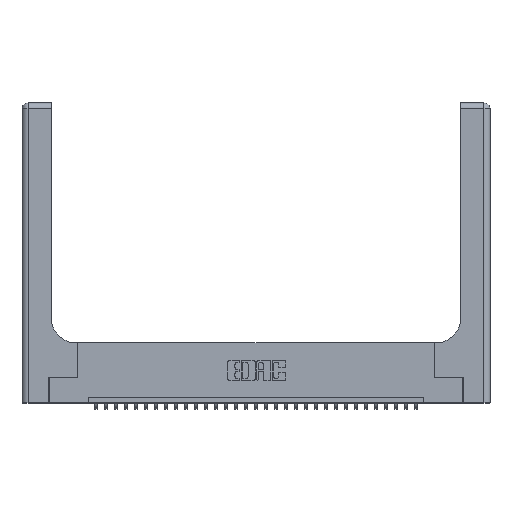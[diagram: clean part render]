
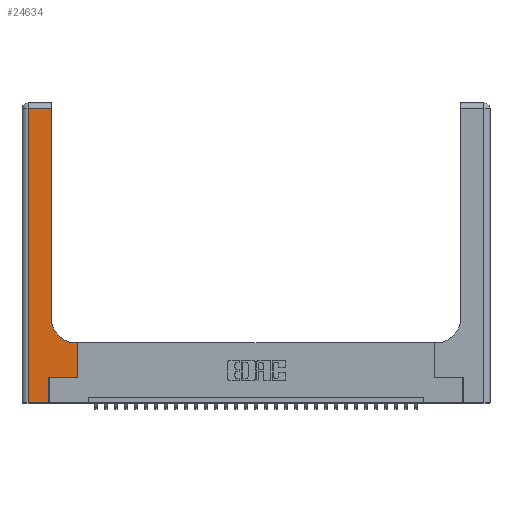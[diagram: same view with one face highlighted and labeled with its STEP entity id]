
A CAD part, top view. The second image highlights one B-rep face of the part: STEP entity #24634.
In plain terms, the highlighted planar face has unit normal (0, 0, 1).
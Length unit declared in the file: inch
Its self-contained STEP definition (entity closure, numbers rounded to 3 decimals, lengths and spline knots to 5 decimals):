
#77 = VERTEX_POINT ( 'NONE', #18571 ) ;
#371 = VECTOR ( 'NONE', #17619, 39.37008 ) ;
#860 = VECTOR ( 'NONE', #27896, 39.37008 ) ;
#1124 = LINE ( 'NONE', #12731, #371 ) ;
#2771 = VECTOR ( 'NONE', #21367, 39.37008 ) ;
#2856 = ORIENTED_EDGE ( 'NONE', *, *, #28152, .T. ) ;
#3835 = DIRECTION ( 'NONE',  ( 1., 0., 0. ) ) ;
#3898 = AXIS2_PLACEMENT_3D ( 'NONE', #25846, #25738, #23431 ) ;
#4235 = VECTOR ( 'NONE', #31249, 39.37008 ) ;
#4257 = ORIENTED_EDGE ( 'NONE', *, *, #28473, .T. ) ;
#4425 = CARTESIAN_POINT ( 'NONE',  ( 0.5415, 0.6, 0.37 ) ) ;
#5604 = ORIENTED_EDGE ( 'NONE', *, *, #16896, .T. ) ;
#5617 = AXIS2_PLACEMENT_3D ( 'NONE', #22779, #8044, #5933 ) ;
#5933 = DIRECTION ( 'NONE',  ( -1., 0., 0. ) ) ;
#6638 = ORIENTED_EDGE ( 'NONE', *, *, #18883, .T. ) ;
#7008 = LINE ( 'NONE', #28454, #16888 ) ;
#7101 = CARTESIAN_POINT ( 'NONE',  ( 0.2915, 3., 0.37 ) ) ;
#8044 = DIRECTION ( 'NONE',  ( 0., 0., -1. ) ) ;
#8745 = CARTESIAN_POINT ( 'NONE',  ( 0., 0., 0.37 ) ) ;
#9005 = ORIENTED_EDGE ( 'NONE', *, *, #16906, .T. ) ;
#9894 = LINE ( 'NONE', #28218, #2771 ) ;
#9935 = ORIENTED_EDGE ( 'NONE', *, *, #11851, .T. ) ;
#10316 = LINE ( 'NONE', #16171, #860 ) ;
#10802 = EDGE_CURVE ( 'NONE', #11875, #19676, #9894, .T. ) ;
#11637 = DIRECTION ( 'NONE',  ( 0., -1., 0. ) ) ;
#11851 = EDGE_CURVE ( 'NONE', #18672, #19126, #17059, .T. ) ;
#11875 = VERTEX_POINT ( 'NONE', #30527 ) ;
#11893 = VECTOR ( 'NONE', #11637, 39.37008 ) ;
#12731 = CARTESIAN_POINT ( 'NONE',  ( 0.5585, 0.25, 0.37 ) ) ;
#13619 = VECTOR ( 'NONE', #3835, 39.37008 ) ;
#13732 = VERTEX_POINT ( 'NONE', #4425 ) ;
#13745 = VERTEX_POINT ( 'NONE', #18265 ) ;
#13988 = DIRECTION ( 'NONE',  ( 0., 1., 0. ) ) ;
#16171 = CARTESIAN_POINT ( 'NONE',  ( 0., 2.94, 0.37 ) ) ;
#16888 = VECTOR ( 'NONE', #13988, 39.37008 ) ;
#16896 = EDGE_CURVE ( 'NONE', #19126, #11875, #7008, .T. ) ;
#16906 = EDGE_CURVE ( 'NONE', #25138, #18672, #23685, .T. ) ;
#17059 = LINE ( 'NONE', #8745, #13619 ) ;
#17619 = DIRECTION ( 'NONE',  ( 0., 1., 0. ) ) ;
#18031 = LINE ( 'NONE', #7101, #24487 ) ;
#18265 = CARTESIAN_POINT ( 'NONE',  ( 0.5585, 0.6, 0.37 ) ) ;
#18513 = CARTESIAN_POINT ( 'NONE',  ( 0.06, 0., 0.37 ) ) ;
#18571 = CARTESIAN_POINT ( 'NONE',  ( 0.2915, 0.85, 0.37 ) ) ;
#18608 = LINE ( 'NONE', #21775, #4235 ) ;
#18672 = VERTEX_POINT ( 'NONE', #18513 ) ;
#18883 = EDGE_CURVE ( 'NONE', #13745, #13732, #18608, .T. ) ;
#19126 = VERTEX_POINT ( 'NONE', #28166 ) ;
#19225 = ORIENTED_EDGE ( 'NONE', *, *, #30047, .T. ) ;
#19585 = CIRCLE ( 'NONE', #3898, 0.25 ) ;
#19676 = VERTEX_POINT ( 'NONE', #30096 ) ;
#19957 = ORIENTED_EDGE ( 'NONE', *, *, #20204, .T. ) ;
#20204 = EDGE_CURVE ( 'NONE', #19676, #13745, #1124, .T. ) ;
#21367 = DIRECTION ( 'NONE',  ( 1., 0., 0. ) ) ;
#21595 = ORIENTED_EDGE ( 'NONE', *, *, #10802, .T. ) ;
#21715 = DIRECTION ( 'NONE',  ( 0., 1., 0. ) ) ;
#21775 = CARTESIAN_POINT ( 'NONE',  ( 0.2915, 0.6, 0.37 ) ) ;
#22623 = CARTESIAN_POINT ( 'NONE',  ( 0.06, 2.94, 0.37 ) ) ;
#22779 = CARTESIAN_POINT ( 'NONE',  ( 0., 3., 0.37 ) ) ;
#23431 = DIRECTION ( 'NONE',  ( 1., 0., 0. ) ) ;
#23525 = EDGE_LOOP ( 'NONE', ( #4257, #19225, #9005, #9935, #5604, #21595, #19957, #6638, #2856 ) ) ;
#23685 = LINE ( 'NONE', #23743, #11893 ) ;
#23743 = CARTESIAN_POINT ( 'NONE',  ( 0.06, 3., 0.37 ) ) ;
#24077 = FACE_OUTER_BOUND ( 'NONE', #23525, .T. ) ;
#24487 = VECTOR ( 'NONE', #21715, 39.37008 ) ;
#24634 = ADVANCED_FACE ( 'NONE', ( #24077 ), #29814, .F. ) ;
#25138 = VERTEX_POINT ( 'NONE', #22623 ) ;
#25738 = DIRECTION ( 'NONE',  ( 0., 0., -1. ) ) ;
#25846 = CARTESIAN_POINT ( 'NONE',  ( 0.5415, 0.85, 0.37 ) ) ;
#27896 = DIRECTION ( 'NONE',  ( -1., 0., 0. ) ) ;
#28152 = EDGE_CURVE ( 'NONE', #13732, #77, #19585, .T. ) ;
#28166 = CARTESIAN_POINT ( 'NONE',  ( 0.269, 0., 0.37 ) ) ;
#28218 = CARTESIAN_POINT ( 'NONE',  ( 0.269, 0.25, 0.37 ) ) ;
#28424 = VERTEX_POINT ( 'NONE', #31097 ) ;
#28454 = CARTESIAN_POINT ( 'NONE',  ( 0.269, 0., 0.37 ) ) ;
#28473 = EDGE_CURVE ( 'NONE', #77, #28424, #18031, .T. ) ;
#29814 = PLANE ( 'NONE',  #5617 ) ;
#30047 = EDGE_CURVE ( 'NONE', #28424, #25138, #10316, .T. ) ;
#30096 = CARTESIAN_POINT ( 'NONE',  ( 0.5585, 0.25, 0.37 ) ) ;
#30527 = CARTESIAN_POINT ( 'NONE',  ( 0.269, 0.25, 0.37 ) ) ;
#31097 = CARTESIAN_POINT ( 'NONE',  ( 0.2915, 2.94, 0.37 ) ) ;
#31249 = DIRECTION ( 'NONE',  ( -1., 0., 0. ) ) ;
